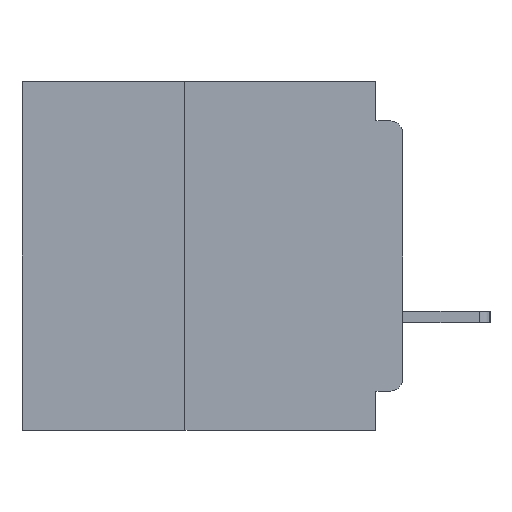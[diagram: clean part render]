
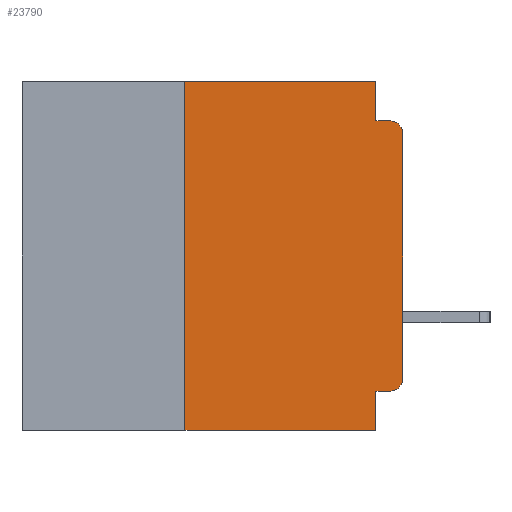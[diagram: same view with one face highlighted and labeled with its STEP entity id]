
A CAD part, left-side view. The second image highlights one B-rep face of the part: STEP entity #23790.
In plain terms, the highlighted planar face has unit normal (-1, 0, 0).
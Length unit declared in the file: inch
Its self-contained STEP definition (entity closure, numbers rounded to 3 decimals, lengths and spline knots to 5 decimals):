
#525 = CIRCLE ( 'NONE', #26691, 0.015 ) ;
#1132 = DIRECTION ( 'NONE',  ( -1., 0., 0. ) ) ;
#1143 = ORIENTED_EDGE ( 'NONE', *, *, #58865, .F. ) ;
#2352 = LINE ( 'NONE', #29513, #42917 ) ;
#3441 = CARTESIAN_POINT ( 'NONE',  ( 0., 0.015, -0.34 ) ) ;
#3713 = VERTEX_POINT ( 'NONE', #24374 ) ;
#5223 = ORIENTED_EDGE ( 'NONE', *, *, #29896, .T. ) ;
#5647 = VECTOR ( 'NONE', #35623, 39.37008 ) ;
#6658 = CARTESIAN_POINT ( 'NONE',  ( 0., 0., -0.355 ) ) ;
#7620 = VECTOR ( 'NONE', #29503, 39.37008 ) ;
#8517 = ORIENTED_EDGE ( 'NONE', *, *, #58677, .F. ) ;
#8656 = CARTESIAN_POINT ( 'NONE',  ( 0., 0.437, -0.4 ) ) ;
#8789 = DIRECTION ( 'NONE',  ( 0., 0., -1. ) ) ;
#8967 = DIRECTION ( 'NONE',  ( 1., 0., 0. ) ) ;
#10129 = CARTESIAN_POINT ( 'NONE',  ( 0., 0.031, -0.4 ) ) ;
#10614 = ORIENTED_EDGE ( 'NONE', *, *, #39481, .T. ) ;
#10942 = ORIENTED_EDGE ( 'NONE', *, *, #52592, .F. ) ;
#12502 = CARTESIAN_POINT ( 'NONE',  ( 0., 0., 0. ) ) ;
#13030 = VERTEX_POINT ( 'NONE', #43022 ) ;
#13599 = DIRECTION ( 'NONE',  ( 0., 0., 1. ) ) ;
#14683 = ORIENTED_EDGE ( 'NONE', *, *, #57974, .T. ) ;
#14837 = DIRECTION ( 'NONE',  ( 0., -1., 0. ) ) ;
#15138 = EDGE_CURVE ( 'NONE', #13030, #37189, #41867, .T. ) ;
#15711 = VECTOR ( 'NONE', #33441, 39.37008 ) ;
#16380 = VERTEX_POINT ( 'NONE', #22556 ) ;
#17185 = ORIENTED_EDGE ( 'NONE', *, *, #31588, .F. ) ;
#17380 = LINE ( 'NONE', #28171, #15711 ) ;
#19458 = PLANE ( 'NONE',  #48376 ) ;
#20914 = VERTEX_POINT ( 'NONE', #27270 ) ;
#21517 = EDGE_LOOP ( 'NONE', ( #57946, #14683, #67383, #8517, #17185, #1143, #5223, #10942, #32167, #10614 ) ) ;
#21521 = LINE ( 'NONE', #51498, #5647 ) ;
#22163 = VERTEX_POINT ( 'NONE', #33765 ) ;
#22287 = VERTEX_POINT ( 'NONE', #34915 ) ;
#22556 = CARTESIAN_POINT ( 'NONE',  ( 0., 0.015, -0.045 ) ) ;
#23790 = ADVANCED_FACE ( 'NONE', ( #48055 ), #19458, .F. ) ;
#24374 = CARTESIAN_POINT ( 'NONE',  ( 0., 0.25, -0.4 ) ) ;
#25969 = EDGE_CURVE ( 'NONE', #20914, #66250, #43720, .T. ) ;
#26691 = AXIS2_PLACEMENT_3D ( 'NONE', #3441, #40475, #8789 ) ;
#27270 = CARTESIAN_POINT ( 'NONE',  ( 0., 0., -0.34 ) ) ;
#28171 = CARTESIAN_POINT ( 'NONE',  ( 0., 0.031, 0. ) ) ;
#29466 = VERTEX_POINT ( 'NONE', #10129 ) ;
#29503 = DIRECTION ( 'NONE',  ( 0., -1., 0. ) ) ;
#29513 = CARTESIAN_POINT ( 'NONE',  ( 0., 0.25, -0.4 ) ) ;
#29896 = EDGE_CURVE ( 'NONE', #3713, #29466, #59032, .T. ) ;
#30510 = CARTESIAN_POINT ( 'NONE',  ( 0., 0., -0.045 ) ) ;
#31062 = VECTOR ( 'NONE', #61391, 39.37008 ) ;
#31588 = EDGE_CURVE ( 'NONE', #22163, #44667, #34096, .T. ) ;
#32167 = ORIENTED_EDGE ( 'NONE', *, *, #15138, .F. ) ;
#32839 = CARTESIAN_POINT ( 'NONE',  ( 0., 0.015, -0.06 ) ) ;
#33441 = DIRECTION ( 'NONE',  ( 0., 0., -1. ) ) ;
#33765 = CARTESIAN_POINT ( 'NONE',  ( 0., 0.25, 0. ) ) ;
#33950 = CIRCLE ( 'NONE', #38068, 0.015 ) ;
#34096 = LINE ( 'NONE', #45461, #7620 ) ;
#34915 = CARTESIAN_POINT ( 'NONE',  ( 0., 0.031, -0.045 ) ) ;
#35623 = DIRECTION ( 'NONE',  ( 0., 0., -1. ) ) ;
#36240 = LINE ( 'NONE', #30510, #48589 ) ;
#36922 = VECTOR ( 'NONE', #54234, 39.37008 ) ;
#37189 = VERTEX_POINT ( 'NONE', #57145 ) ;
#38068 = AXIS2_PLACEMENT_3D ( 'NONE', #32839, #1132, #38194 ) ;
#38194 = DIRECTION ( 'NONE',  ( 0., 0., -1. ) ) ;
#38820 = DIRECTION ( 'NONE',  ( 0., 0., 1. ) ) ;
#39481 = EDGE_CURVE ( 'NONE', #13030, #20914, #525, .T. ) ;
#40475 = DIRECTION ( 'NONE',  ( -1., 0., 0. ) ) ;
#40655 = CARTESIAN_POINT ( 'NONE',  ( 0., 0.437, 0. ) ) ;
#41264 = CARTESIAN_POINT ( 'NONE',  ( 0., 0., -0.06 ) ) ;
#41428 = EDGE_CURVE ( 'NONE', #22287, #16380, #36240, .T. ) ;
#41867 = LINE ( 'NONE', #6658, #36922 ) ;
#42917 = VECTOR ( 'NONE', #13599, 39.37008 ) ;
#43022 = CARTESIAN_POINT ( 'NONE',  ( 0., 0.015, -0.355 ) ) ;
#43720 = LINE ( 'NONE', #12502, #56041 ) ;
#44667 = VERTEX_POINT ( 'NONE', #63258 ) ;
#45461 = CARTESIAN_POINT ( 'NONE',  ( 0., 0.437, 0. ) ) ;
#45962 = DIRECTION ( 'NONE',  ( 0., 0., -1. ) ) ;
#48055 = FACE_OUTER_BOUND ( 'NONE', #21517, .T. ) ;
#48376 = AXIS2_PLACEMENT_3D ( 'NONE', #40655, #8967, #45962 ) ;
#48589 = VECTOR ( 'NONE', #14837, 39.37008 ) ;
#51498 = CARTESIAN_POINT ( 'NONE',  ( 0., 0.031, -0.4 ) ) ;
#52592 = EDGE_CURVE ( 'NONE', #37189, #29466, #21521, .T. ) ;
#54234 = DIRECTION ( 'NONE',  ( 0., 1., 0. ) ) ;
#56041 = VECTOR ( 'NONE', #38820, 39.37008 ) ;
#57145 = CARTESIAN_POINT ( 'NONE',  ( 0., 0.031, -0.355 ) ) ;
#57946 = ORIENTED_EDGE ( 'NONE', *, *, #25969, .T. ) ;
#57974 = EDGE_CURVE ( 'NONE', #66250, #16380, #33950, .T. ) ;
#58677 = EDGE_CURVE ( 'NONE', #44667, #22287, #17380, .T. ) ;
#58865 = EDGE_CURVE ( 'NONE', #3713, #22163, #2352, .T. ) ;
#59032 = LINE ( 'NONE', #8656, #31062 ) ;
#61391 = DIRECTION ( 'NONE',  ( 0., -1., 0. ) ) ;
#63258 = CARTESIAN_POINT ( 'NONE',  ( 0., 0.031, 0. ) ) ;
#66250 = VERTEX_POINT ( 'NONE', #41264 ) ;
#67383 = ORIENTED_EDGE ( 'NONE', *, *, #41428, .F. ) ;
